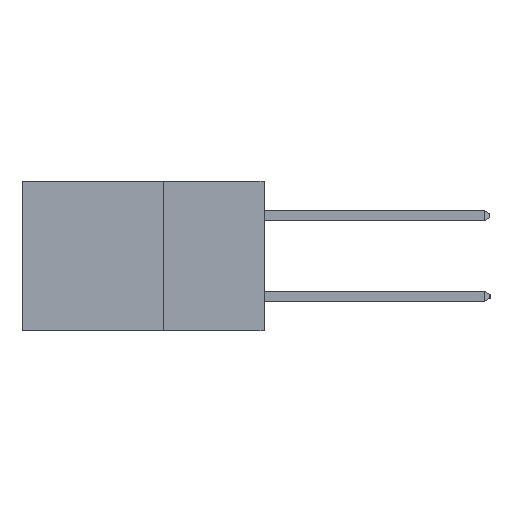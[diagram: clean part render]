
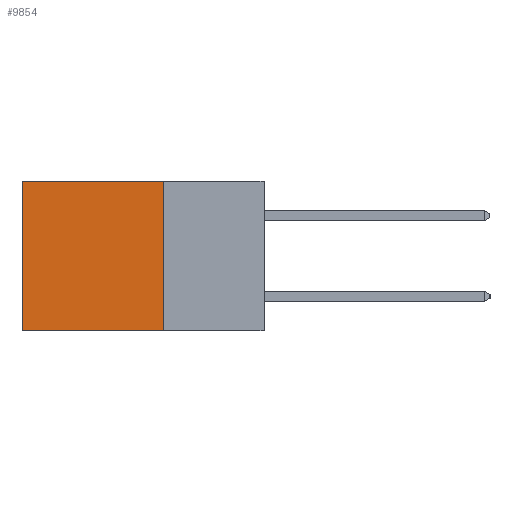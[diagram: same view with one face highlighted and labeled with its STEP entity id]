
A CAD part, left-side view. The second image highlights one B-rep face of the part: STEP entity #9854.
In plain terms, the highlighted planar face has unit normal (-1, 0, 0).
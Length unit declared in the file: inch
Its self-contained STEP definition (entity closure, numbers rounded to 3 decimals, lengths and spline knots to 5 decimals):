
#49 = EDGE_CURVE ( 'NONE', #6925, #1214, #5706, .T. ) ;
#125 = VERTEX_POINT ( 'NONE', #2214 ) ;
#584 = VECTOR ( 'NONE', #6967, 39.37008 ) ;
#1040 = LINE ( 'NONE', #2252, #10507 ) ;
#1092 = AXIS2_PLACEMENT_3D ( 'NONE', #11867, #10953, #10941 ) ;
#1214 = VERTEX_POINT ( 'NONE', #9374 ) ;
#2174 = EDGE_LOOP ( 'NONE', ( #4742, #2381, #4510, #6292 ) ) ;
#2184 = DIRECTION ( 'NONE',  ( 0., 1., 0. ) ) ;
#2214 = CARTESIAN_POINT ( 'NONE',  ( 0.2615, 0.6, 0. ) ) ;
#2252 = CARTESIAN_POINT ( 'NONE',  ( 0.2615, 0.25, 0. ) ) ;
#2381 = ORIENTED_EDGE ( 'NONE', *, *, #5494, .F. ) ;
#2449 = CARTESIAN_POINT ( 'NONE',  ( 0.2615, 0.6, -0.37 ) ) ;
#2593 = LINE ( 'NONE', #2449, #2888 ) ;
#2859 = DIRECTION ( 'NONE',  ( 0., 0., -1. ) ) ;
#2888 = VECTOR ( 'NONE', #2859, 39.37008 ) ;
#3044 = FACE_OUTER_BOUND ( 'NONE', #2174, .T. ) ;
#4171 = EDGE_CURVE ( 'NONE', #125, #11423, #2593, .T. ) ;
#4510 = ORIENTED_EDGE ( 'NONE', *, *, #49, .F. ) ;
#4742 = ORIENTED_EDGE ( 'NONE', *, *, #4171, .T. ) ;
#5421 = VECTOR ( 'NONE', #6085, 39.37008 ) ;
#5494 = EDGE_CURVE ( 'NONE', #1214, #11423, #7916, .T. ) ;
#5706 = LINE ( 'NONE', #11855, #584 ) ;
#6085 = DIRECTION ( 'NONE',  ( 0., 1., 0. ) ) ;
#6167 = EDGE_CURVE ( 'NONE', #6925, #125, #1040, .T. ) ;
#6219 = CARTESIAN_POINT ( 'NONE',  ( 0.2615, 0.25, -0.37 ) ) ;
#6292 = ORIENTED_EDGE ( 'NONE', *, *, #6167, .T. ) ;
#6925 = VERTEX_POINT ( 'NONE', #9025 ) ;
#6967 = DIRECTION ( 'NONE',  ( 0., 0., -1. ) ) ;
#7916 = LINE ( 'NONE', #6219, #5421 ) ;
#9025 = CARTESIAN_POINT ( 'NONE',  ( 0.2615, 0.25, 0. ) ) ;
#9374 = CARTESIAN_POINT ( 'NONE',  ( 0.2615, 0.25, -0.37 ) ) ;
#9854 = ADVANCED_FACE ( 'NONE', ( #3044 ), #11139, .F. ) ;
#10507 = VECTOR ( 'NONE', #2184, 39.37008 ) ;
#10941 = DIRECTION ( 'NONE',  ( 0., 0., -1. ) ) ;
#10953 = DIRECTION ( 'NONE',  ( 1., 0., 0. ) ) ;
#11139 = PLANE ( 'NONE',  #1092 ) ;
#11174 = CARTESIAN_POINT ( 'NONE',  ( 0.2615, 0.6, -0.37 ) ) ;
#11423 = VERTEX_POINT ( 'NONE', #11174 ) ;
#11855 = CARTESIAN_POINT ( 'NONE',  ( 0.2615, 0.25, -0.37 ) ) ;
#11867 = CARTESIAN_POINT ( 'NONE',  ( 0.2615, 0.25, -0.37 ) ) ;
